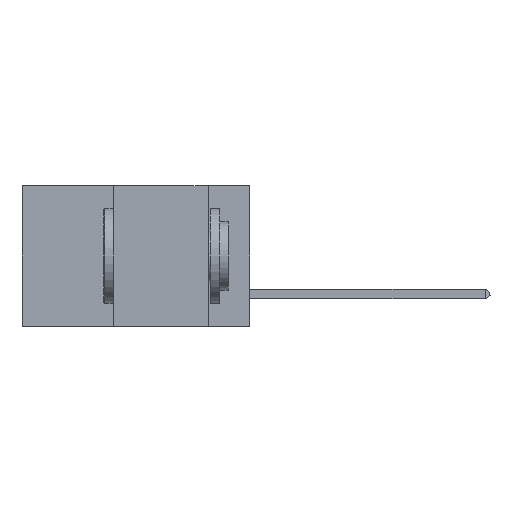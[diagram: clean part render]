
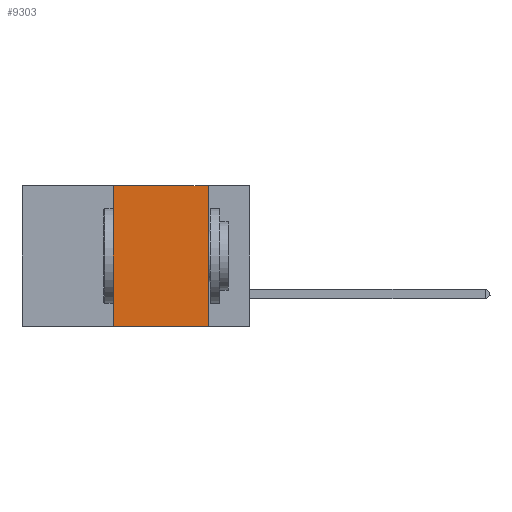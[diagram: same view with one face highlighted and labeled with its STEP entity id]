
A CAD part, left-side view. The second image highlights one B-rep face of the part: STEP entity #9303.
In plain terms, the highlighted planar face has unit normal (-1, 0, 0).
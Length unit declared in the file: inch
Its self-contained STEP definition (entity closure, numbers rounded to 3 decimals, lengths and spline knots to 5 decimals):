
#1303 = LINE ( 'NONE', #3346, #5518 ) ;
#1451 = CARTESIAN_POINT ( 'NONE',  ( 0., 0.11, 0. ) ) ;
#1454 = EDGE_CURVE ( 'NONE', #5892, #3239, #1303, .T. ) ;
#1499 = DIRECTION ( 'NONE',  ( 0., -1., 0. ) ) ;
#2506 = DIRECTION ( 'NONE',  ( 0., -1., 0. ) ) ;
#2627 = AXIS2_PLACEMENT_3D ( 'NONE', #6075, #7943, #7982 ) ;
#2677 = CARTESIAN_POINT ( 'NONE',  ( 0., 0.6, -0.37 ) ) ;
#3239 = VERTEX_POINT ( 'NONE', #5959 ) ;
#3346 = CARTESIAN_POINT ( 'NONE',  ( 0., 0.6, 0. ) ) ;
#3412 = EDGE_CURVE ( 'NONE', #3239, #11033, #11592, .T. ) ;
#3610 = ORIENTED_EDGE ( 'NONE', *, *, #1454, .F. ) ;
#3735 = DIRECTION ( 'NONE',  ( 0., 0., 1. ) ) ;
#3968 = EDGE_LOOP ( 'NONE', ( #11845, #3610, #9973, #5063 ) ) ;
#4174 = CARTESIAN_POINT ( 'NONE',  ( 0., 0.11, -0.37 ) ) ;
#4249 = DIRECTION ( 'NONE',  ( 0., 0., -1. ) ) ;
#4289 = PLANE ( 'NONE',  #2627 ) ;
#4623 = LINE ( 'NONE', #2677, #8364 ) ;
#4798 = EDGE_CURVE ( 'NONE', #6323, #5892, #9775, .T. ) ;
#5063 = ORIENTED_EDGE ( 'NONE', *, *, #5098, .T. ) ;
#5090 = CARTESIAN_POINT ( 'NONE',  ( 0., 0.36, 0. ) ) ;
#5098 = EDGE_CURVE ( 'NONE', #6323, #11033, #4623, .T. ) ;
#5158 = VECTOR ( 'NONE', #4249, 39.37008 ) ;
#5518 = VECTOR ( 'NONE', #1499, 39.37008 ) ;
#5892 = VERTEX_POINT ( 'NONE', #5090 ) ;
#5959 = CARTESIAN_POINT ( 'NONE',  ( 0., 0.11, 0. ) ) ;
#6075 = CARTESIAN_POINT ( 'NONE',  ( 0., 0.6, 0. ) ) ;
#6323 = VERTEX_POINT ( 'NONE', #9340 ) ;
#6738 = VECTOR ( 'NONE', #3735, 39.37008 ) ;
#7943 = DIRECTION ( 'NONE',  ( 1., 0., 0. ) ) ;
#7982 = DIRECTION ( 'NONE',  ( 0., 0., -1. ) ) ;
#8364 = VECTOR ( 'NONE', #2506, 39.37008 ) ;
#9164 = CARTESIAN_POINT ( 'NONE',  ( 0., 0.36, 0. ) ) ;
#9303 = ADVANCED_FACE ( 'NONE', ( #10152 ), #4289, .F. ) ;
#9340 = CARTESIAN_POINT ( 'NONE',  ( 0., 0.36, -0.37 ) ) ;
#9775 = LINE ( 'NONE', #9164, #6738 ) ;
#9973 = ORIENTED_EDGE ( 'NONE', *, *, #4798, .F. ) ;
#10152 = FACE_OUTER_BOUND ( 'NONE', #3968, .T. ) ;
#11033 = VERTEX_POINT ( 'NONE', #4174 ) ;
#11592 = LINE ( 'NONE', #1451, #5158 ) ;
#11845 = ORIENTED_EDGE ( 'NONE', *, *, #3412, .F. ) ;
